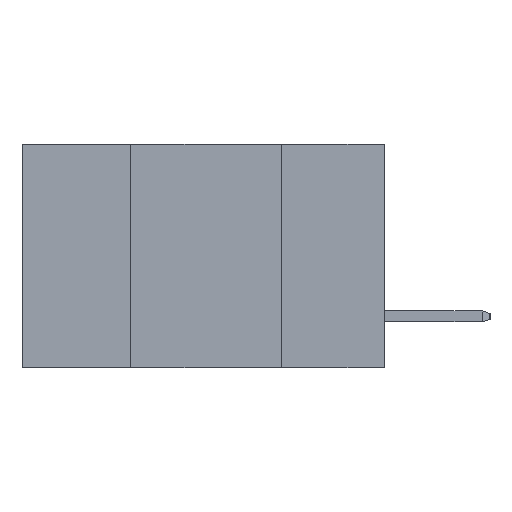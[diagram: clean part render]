
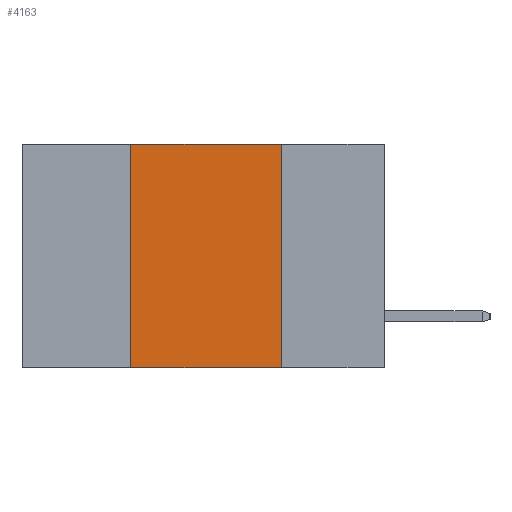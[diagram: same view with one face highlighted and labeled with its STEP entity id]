
A CAD part, left-side view. The second image highlights one B-rep face of the part: STEP entity #4163.
In plain terms, the highlighted planar face has unit normal (-1, 0, 0).
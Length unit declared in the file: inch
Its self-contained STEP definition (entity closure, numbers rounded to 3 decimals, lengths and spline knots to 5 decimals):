
#516 = DIRECTION ( 'NONE',  ( 0., 0., -1. ) ) ;
#662 = EDGE_CURVE ( 'NONE', #1757, #7593, #1059, .T. ) ;
#721 = DIRECTION ( 'NONE',  ( 1., 0., 0. ) ) ;
#737 = CARTESIAN_POINT ( 'NONE',  ( 0., 0.6, 0. ) ) ;
#1059 = LINE ( 'NONE', #8016, #10764 ) ;
#1704 = ORIENTED_EDGE ( 'NONE', *, *, #7975, .T. ) ;
#1757 = VERTEX_POINT ( 'NONE', #9050 ) ;
#1918 = PLANE ( 'NONE',  #8108 ) ;
#1981 = VECTOR ( 'NONE', #5891, 39.37008 ) ;
#3154 = CARTESIAN_POINT ( 'NONE',  ( 0., 0.42, 0. ) ) ;
#3930 = FACE_OUTER_BOUND ( 'NONE', #9023, .T. ) ;
#4008 = ORIENTED_EDGE ( 'NONE', *, *, #11585, .F. ) ;
#4163 = ADVANCED_FACE ( 'NONE', ( #3930 ), #1918, .F. ) ;
#4166 = VECTOR ( 'NONE', #10524, 39.37008 ) ;
#4182 = VERTEX_POINT ( 'NONE', #3154 ) ;
#5195 = VERTEX_POINT ( 'NONE', #8971 ) ;
#5850 = CARTESIAN_POINT ( 'NONE',  ( 0., 0.6, 0. ) ) ;
#5871 = VECTOR ( 'NONE', #11741, 39.37008 ) ;
#5891 = DIRECTION ( 'NONE',  ( 0., -1., 0. ) ) ;
#6546 = ORIENTED_EDGE ( 'NONE', *, *, #10407, .F. ) ;
#7083 = LINE ( 'NONE', #5850, #1981 ) ;
#7593 = VERTEX_POINT ( 'NONE', #8430 ) ;
#7661 = DIRECTION ( 'NONE',  ( 0., 0., -1. ) ) ;
#7975 = EDGE_CURVE ( 'NONE', #5195, #7593, #8596, .T. ) ;
#8016 = CARTESIAN_POINT ( 'NONE',  ( 0., 0.17, -0.37 ) ) ;
#8108 = AXIS2_PLACEMENT_3D ( 'NONE', #737, #721, #516 ) ;
#8430 = CARTESIAN_POINT ( 'NONE',  ( 0., 0.17, -0.37 ) ) ;
#8596 = LINE ( 'NONE', #10845, #5871 ) ;
#8971 = CARTESIAN_POINT ( 'NONE',  ( 0., 0.42, -0.37 ) ) ;
#9023 = EDGE_LOOP ( 'NONE', ( #11047, #4008, #6546, #1704 ) ) ;
#9050 = CARTESIAN_POINT ( 'NONE',  ( 0., 0.17, 0. ) ) ;
#9110 = LINE ( 'NONE', #11412, #4166 ) ;
#10407 = EDGE_CURVE ( 'NONE', #5195, #4182, #9110, .T. ) ;
#10524 = DIRECTION ( 'NONE',  ( 0., 0., 1. ) ) ;
#10764 = VECTOR ( 'NONE', #7661, 39.37008 ) ;
#10845 = CARTESIAN_POINT ( 'NONE',  ( 0., 0.6, -0.37 ) ) ;
#11047 = ORIENTED_EDGE ( 'NONE', *, *, #662, .F. ) ;
#11412 = CARTESIAN_POINT ( 'NONE',  ( 0., 0.42, -0.37 ) ) ;
#11585 = EDGE_CURVE ( 'NONE', #4182, #1757, #7083, .T. ) ;
#11741 = DIRECTION ( 'NONE',  ( 0., -1., 0. ) ) ;
